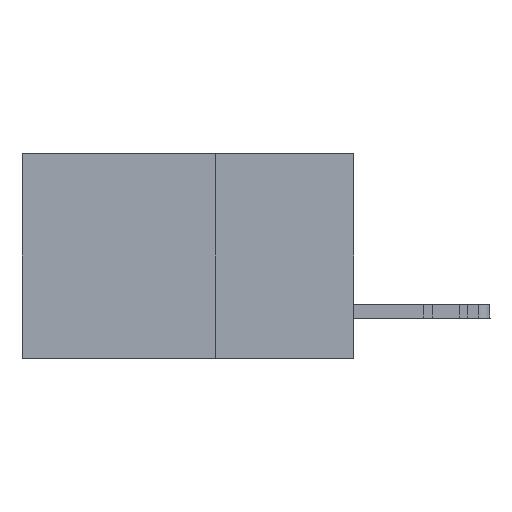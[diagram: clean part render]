
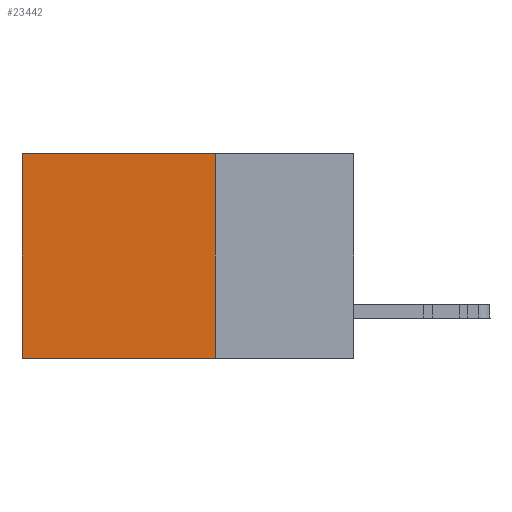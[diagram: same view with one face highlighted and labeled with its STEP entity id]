
A CAD part, left-side view. The second image highlights one B-rep face of the part: STEP entity #23442.
In plain terms, the highlighted planar face has unit normal (-1, 0, 0).
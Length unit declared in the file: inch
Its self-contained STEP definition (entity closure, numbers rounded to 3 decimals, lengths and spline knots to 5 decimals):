
#219 = ORIENTED_EDGE ( 'NONE', *, *, #23223, .T. ) ;
#368 = LINE ( 'NONE', #530, #28180 ) ;
#530 = CARTESIAN_POINT ( 'NONE',  ( 0.2875, 0.25, 0. ) ) ;
#1850 = EDGE_CURVE ( 'NONE', #44446, #14425, #38929, .T. ) ;
#2128 = VECTOR ( 'NONE', #29385, 39.37008 ) ;
#3091 = CARTESIAN_POINT ( 'NONE',  ( 0.2875, 0.25, 0. ) ) ;
#3729 = DIRECTION ( 'NONE',  ( 0., 0., -1. ) ) ;
#3765 = ORIENTED_EDGE ( 'NONE', *, *, #10013, .T. ) ;
#4905 = EDGE_CURVE ( 'NONE', #8093, #44446, #368, .T. ) ;
#8031 = DIRECTION ( 'NONE',  ( 0., 0., -1. ) ) ;
#8093 = VERTEX_POINT ( 'NONE', #46221 ) ;
#10013 = EDGE_CURVE ( 'NONE', #8093, #33780, #17514, .T. ) ;
#10254 = DIRECTION ( 'NONE',  ( 1., 0., 0. ) ) ;
#10454 = ORIENTED_EDGE ( 'NONE', *, *, #4905, .F. ) ;
#14425 = VERTEX_POINT ( 'NONE', #29638 ) ;
#15294 = CARTESIAN_POINT ( 'NONE',  ( 0.2875, 0.25, -0.37 ) ) ;
#15825 = LINE ( 'NONE', #19600, #33872 ) ;
#17514 = LINE ( 'NONE', #17788, #40185 ) ;
#17788 = CARTESIAN_POINT ( 'NONE',  ( 0.2875, 0.25, 0. ) ) ;
#17944 = DIRECTION ( 'NONE',  ( 0., 1., 0. ) ) ;
#19600 = CARTESIAN_POINT ( 'NONE',  ( 0.2875, 0.6, 0. ) ) ;
#19643 = EDGE_LOOP ( 'NONE', ( #219, #31692, #10454, #3765 ) ) ;
#23223 = EDGE_CURVE ( 'NONE', #33780, #14425, #15825, .T. ) ;
#23442 = ADVANCED_FACE ( 'NONE', ( #45748 ), #24804, .F. ) ;
#24804 = PLANE ( 'NONE',  #25239 ) ;
#25239 = AXIS2_PLACEMENT_3D ( 'NONE', #3091, #10254, #39195 ) ;
#28180 = VECTOR ( 'NONE', #3729, 39.37008 ) ;
#29240 = CARTESIAN_POINT ( 'NONE',  ( 0.2875, 0.25, -0.37 ) ) ;
#29385 = DIRECTION ( 'NONE',  ( 0., 1., 0. ) ) ;
#29638 = CARTESIAN_POINT ( 'NONE',  ( 0.2875, 0.6, -0.37 ) ) ;
#31539 = CARTESIAN_POINT ( 'NONE',  ( 0.2875, 0.6, 0. ) ) ;
#31692 = ORIENTED_EDGE ( 'NONE', *, *, #1850, .F. ) ;
#33780 = VERTEX_POINT ( 'NONE', #31539 ) ;
#33872 = VECTOR ( 'NONE', #8031, 39.37008 ) ;
#38929 = LINE ( 'NONE', #29240, #2128 ) ;
#39195 = DIRECTION ( 'NONE',  ( 0., 0., -1. ) ) ;
#40185 = VECTOR ( 'NONE', #17944, 39.37008 ) ;
#44446 = VERTEX_POINT ( 'NONE', #15294 ) ;
#45748 = FACE_OUTER_BOUND ( 'NONE', #19643, .T. ) ;
#46221 = CARTESIAN_POINT ( 'NONE',  ( 0.2875, 0.25, 0. ) ) ;
